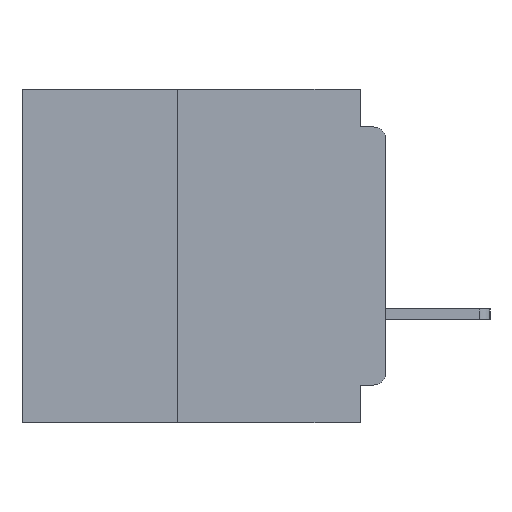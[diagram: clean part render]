
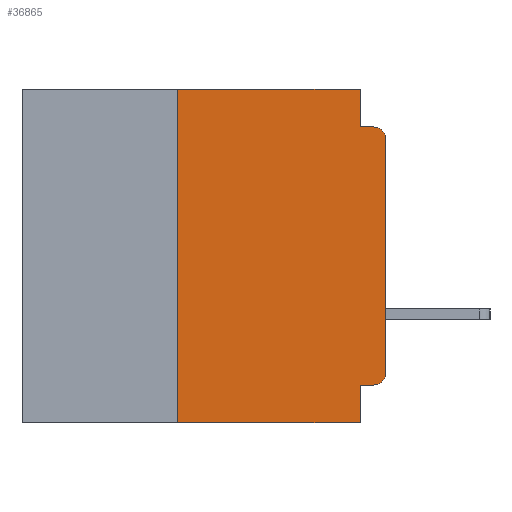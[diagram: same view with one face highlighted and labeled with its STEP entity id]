
A CAD part, left-side view. The second image highlights one B-rep face of the part: STEP entity #36865.
In plain terms, the highlighted planar face has unit normal (-1, 0, 0).
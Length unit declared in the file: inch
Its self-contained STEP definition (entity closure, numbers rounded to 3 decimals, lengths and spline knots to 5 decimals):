
#287 = VERTEX_POINT ( 'NONE', #36081 ) ;
#2226 = CARTESIAN_POINT ( 'NONE',  ( 0., 0., 0. ) ) ;
#3046 = LINE ( 'NONE', #39582, #19006 ) ;
#3635 = VERTEX_POINT ( 'NONE', #9053 ) ;
#3750 = EDGE_CURVE ( 'NONE', #30932, #27419, #6081, .T. ) ;
#4177 = EDGE_CURVE ( 'NONE', #27419, #26468, #39699, .T. ) ;
#4235 = ORIENTED_EDGE ( 'NONE', *, *, #19914, .T. ) ;
#4971 = VERTEX_POINT ( 'NONE', #28493 ) ;
#5387 = DIRECTION ( 'NONE',  ( -1., 0., 0. ) ) ;
#6081 = LINE ( 'NONE', #23171, #30393 ) ;
#6084 = CIRCLE ( 'NONE', #31626, 0.015 ) ;
#7311 = ORIENTED_EDGE ( 'NONE', *, *, #39352, .T. ) ;
#7568 = CARTESIAN_POINT ( 'NONE',  ( 0., 0.437, 0. ) ) ;
#8704 = CARTESIAN_POINT ( 'NONE',  ( 0., 0.25, -0.4 ) ) ;
#8911 = EDGE_CURVE ( 'NONE', #14272, #17031, #34646, .T. ) ;
#9053 = CARTESIAN_POINT ( 'NONE',  ( 0., 0.25, 0. ) ) ;
#9260 = CARTESIAN_POINT ( 'NONE',  ( 0., 0.015, -0.045 ) ) ;
#9423 = LINE ( 'NONE', #9981, #25279 ) ;
#9981 = CARTESIAN_POINT ( 'NONE',  ( 0., 0.437, 0. ) ) ;
#10573 = VECTOR ( 'NONE', #31560, 39.37008 ) ;
#10743 = DIRECTION ( 'NONE',  ( 0., 0., -1. ) ) ;
#11266 = CARTESIAN_POINT ( 'NONE',  ( 0., 0.031, -0.045 ) ) ;
#11838 = DIRECTION ( 'NONE',  ( 0., 0., 1. ) ) ;
#12210 = VECTOR ( 'NONE', #34020, 39.37008 ) ;
#12792 = EDGE_CURVE ( 'NONE', #30450, #287, #15493, .T. ) ;
#12940 = ORIENTED_EDGE ( 'NONE', *, *, #8911, .T. ) ;
#13446 = ORIENTED_EDGE ( 'NONE', *, *, #12792, .F. ) ;
#13669 = EDGE_CURVE ( 'NONE', #17031, #26468, #14420, .T. ) ;
#13770 = EDGE_LOOP ( 'NONE', ( #12940, #15441, #20957, #37268, #17572, #22069, #4235, #13446, #14714, #7311 ) ) ;
#13808 = PLANE ( 'NONE',  #31366 ) ;
#14229 = CARTESIAN_POINT ( 'NONE',  ( 0., 0.015, -0.06 ) ) ;
#14233 = DIRECTION ( 'NONE',  ( 0., 0., -1. ) ) ;
#14272 = VERTEX_POINT ( 'NONE', #17235 ) ;
#14420 = CIRCLE ( 'NONE', #19330, 0.015 ) ;
#14714 = ORIENTED_EDGE ( 'NONE', *, *, #26518, .F. ) ;
#15441 = ORIENTED_EDGE ( 'NONE', *, *, #13669, .T. ) ;
#15493 = LINE ( 'NONE', #36746, #23934 ) ;
#17031 = VERTEX_POINT ( 'NONE', #32318 ) ;
#17235 = CARTESIAN_POINT ( 'NONE',  ( 0., 0., -0.34 ) ) ;
#17416 = DIRECTION ( 'NONE',  ( 0., 0., -1. ) ) ;
#17572 = ORIENTED_EDGE ( 'NONE', *, *, #34779, .F. ) ;
#17862 = VECTOR ( 'NONE', #11838, 39.37008 ) ;
#17962 = EDGE_CURVE ( 'NONE', #4971, #3635, #29084, .T. ) ;
#19006 = VECTOR ( 'NONE', #27032, 39.37008 ) ;
#19330 = AXIS2_PLACEMENT_3D ( 'NONE', #14229, #36325, #17416 ) ;
#19914 = EDGE_CURVE ( 'NONE', #4971, #287, #3046, .T. ) ;
#20957 = ORIENTED_EDGE ( 'NONE', *, *, #4177, .F. ) ;
#22069 = ORIENTED_EDGE ( 'NONE', *, *, #17962, .F. ) ;
#22177 = CARTESIAN_POINT ( 'NONE',  ( 0., 0., -0.355 ) ) ;
#23171 = CARTESIAN_POINT ( 'NONE',  ( 0., 0.031, 0. ) ) ;
#23934 = VECTOR ( 'NONE', #30451, 39.37008 ) ;
#24370 = CARTESIAN_POINT ( 'NONE',  ( 0., 0.015, -0.34 ) ) ;
#25279 = VECTOR ( 'NONE', #35301, 39.37008 ) ;
#26468 = VERTEX_POINT ( 'NONE', #9260 ) ;
#26518 = EDGE_CURVE ( 'NONE', #27852, #30450, #36784, .T. ) ;
#27032 = DIRECTION ( 'NONE',  ( 0., -1., 0. ) ) ;
#27419 = VERTEX_POINT ( 'NONE', #11266 ) ;
#27541 = DIRECTION ( 'NONE',  ( 0., 0., -1. ) ) ;
#27769 = CARTESIAN_POINT ( 'NONE',  ( 0., 0.015, -0.355 ) ) ;
#27852 = VERTEX_POINT ( 'NONE', #27769 ) ;
#28493 = CARTESIAN_POINT ( 'NONE',  ( 0., 0.25, -0.4 ) ) ;
#29084 = LINE ( 'NONE', #8704, #12210 ) ;
#29734 = DIRECTION ( 'NONE',  ( 1., 0., 0. ) ) ;
#30393 = VECTOR ( 'NONE', #14233, 39.37008 ) ;
#30450 = VERTEX_POINT ( 'NONE', #38195 ) ;
#30451 = DIRECTION ( 'NONE',  ( 0., 0., -1. ) ) ;
#30932 = VERTEX_POINT ( 'NONE', #40655 ) ;
#31343 = VECTOR ( 'NONE', #39103, 39.37008 ) ;
#31366 = AXIS2_PLACEMENT_3D ( 'NONE', #7568, #29734, #10743 ) ;
#31560 = DIRECTION ( 'NONE',  ( 0., 1., 0. ) ) ;
#31626 = AXIS2_PLACEMENT_3D ( 'NONE', #24370, #5387, #27541 ) ;
#32318 = CARTESIAN_POINT ( 'NONE',  ( 0., 0., -0.06 ) ) ;
#34020 = DIRECTION ( 'NONE',  ( 0., 0., 1. ) ) ;
#34646 = LINE ( 'NONE', #2226, #17862 ) ;
#34779 = EDGE_CURVE ( 'NONE', #3635, #30932, #9423, .T. ) ;
#35301 = DIRECTION ( 'NONE',  ( 0., -1., 0. ) ) ;
#36031 = FACE_OUTER_BOUND ( 'NONE', #13770, .T. ) ;
#36081 = CARTESIAN_POINT ( 'NONE',  ( 0., 0.031, -0.4 ) ) ;
#36325 = DIRECTION ( 'NONE',  ( -1., 0., 0. ) ) ;
#36746 = CARTESIAN_POINT ( 'NONE',  ( 0., 0.031, -0.4 ) ) ;
#36784 = LINE ( 'NONE', #22177, #10573 ) ;
#36865 = ADVANCED_FACE ( 'NONE', ( #36031 ), #13808, .F. ) ;
#37268 = ORIENTED_EDGE ( 'NONE', *, *, #3750, .F. ) ;
#38195 = CARTESIAN_POINT ( 'NONE',  ( 0., 0.031, -0.355 ) ) ;
#39015 = CARTESIAN_POINT ( 'NONE',  ( 0., 0., -0.045 ) ) ;
#39103 = DIRECTION ( 'NONE',  ( 0., -1., 0. ) ) ;
#39352 = EDGE_CURVE ( 'NONE', #27852, #14272, #6084, .T. ) ;
#39582 = CARTESIAN_POINT ( 'NONE',  ( 0., 0.437, -0.4 ) ) ;
#39699 = LINE ( 'NONE', #39015, #31343 ) ;
#40655 = CARTESIAN_POINT ( 'NONE',  ( 0., 0.031, 0. ) ) ;
